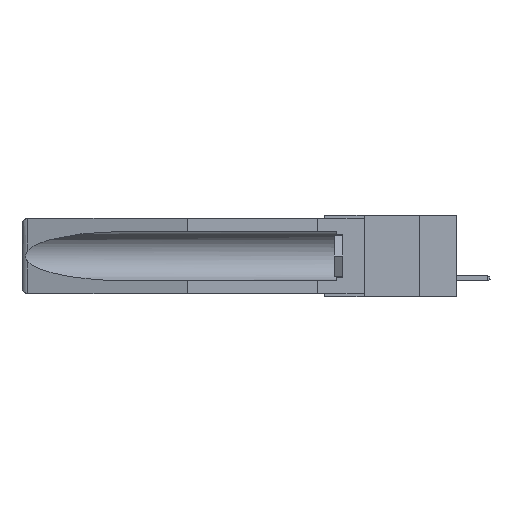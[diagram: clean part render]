
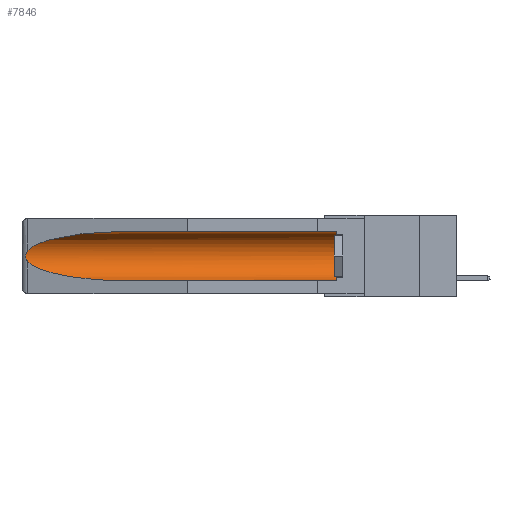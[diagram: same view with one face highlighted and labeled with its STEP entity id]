
A CAD part, left-side view. The second image highlights one B-rep face of the part: STEP entity #7846.
In plain terms, the highlighted cylindrical face has radius 2.857 mm (diameter 5.715 mm), a partial arc.
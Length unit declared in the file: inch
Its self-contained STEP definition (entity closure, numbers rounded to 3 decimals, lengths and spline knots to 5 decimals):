
#14 = CYLINDRICAL_SURFACE ( 'NONE', #1620, 0.1125 ) ;
#582 = CARTESIAN_POINT ( 'NONE',  ( 0.155, -0.30754, -0.284 ) ) ;
#1620 = AXIS2_PLACEMENT_3D ( 'NONE', #8060, #27274, #1698 ) ;
#1633 = CARTESIAN_POINT ( 'NONE',  ( 0.155, 0.126, -0.059 ) ) ;
#1698 = DIRECTION ( 'NONE',  ( 0., 0., 1. ) ) ;
#1851 = CARTESIAN_POINT ( 'NONE',  ( 0.26537, 1.52718, -0.14972 ) ) ;
#2021 = CARTESIAN_POINT ( 'NONE',  ( 0.2675, 1.53308, -0.17534 ) ) ;
#3141 = CARTESIAN_POINT ( 'NONE',  ( 0.26537, 1.52718, -0.19328 ) ) ;
#3952 = CARTESIAN_POINT ( 'NONE',  ( 0.26597, 1.5296, -0.19026 ) ) ;
#4129 = EDGE_CURVE ( 'NONE', #7265, #11339, #20582, .T. ) ;
#4150 = CARTESIAN_POINT ( 'NONE',  ( 0.26537, 1.52718, -0.14972 ) ) ;
#4466 = VERTEX_POINT ( 'NONE', #5350 ) ;
#5350 = CARTESIAN_POINT ( 'NONE',  ( 0.26537, 1.52718, -0.14972 ) ) ;
#5520 = EDGE_CURVE ( 'NONE', #24742, #11339, #21461, .T. ) ;
#6110 = AXIS2_PLACEMENT_3D ( 'NONE', #10909, #21558, #17171 ) ;
#6235 = CARTESIAN_POINT ( 'NONE',  ( 0.26537, 1.52718, -0.19328 ) ) ;
#6676 = ORIENTED_EDGE ( 'NONE', *, *, #16037, .T. ) ;
#6684 = ORIENTED_EDGE ( 'NONE', *, *, #20592, .T. ) ;
#7265 = VERTEX_POINT ( 'NONE', #25943 ) ;
#7846 = ADVANCED_FACE ( 'NONE', ( #17055 ), #14, .F. ) ;
#8060 = CARTESIAN_POINT ( 'NONE',  ( 0.155, -0.30754, -0.1715 ) ) ;
#8116 = DIRECTION ( 'NONE',  ( 0., 1., 0. ) ) ;
#8688 = CARTESIAN_POINT ( 'NONE',  ( 0.155, 1.07973, -0.284 ) ) ;
#9482 =( BOUNDED_CURVE ( )  B_SPLINE_CURVE ( 3, ( #14633, #25220, #20997, #4150 ),
 .UNSPECIFIED., .F., .F. ) 
 B_SPLINE_CURVE_WITH_KNOTS ( ( 4, 4 ),
 ( 4.71239, 6.08839 ),
 .UNSPECIFIED. ) 
 CURVE ( )  GEOMETRIC_REPRESENTATION_ITEM ( )  RATIONAL_B_SPLINE_CURVE ( ( 1., 0.848, 0.848, 1. ) ) 
 REPRESENTATION_ITEM ( '' )  );
#10348 = CARTESIAN_POINT ( 'NONE',  ( 0.155, -0.30754, -0.059 ) ) ;
#10535 = CARTESIAN_POINT ( 'NONE',  ( 0.2673, 1.53269, -0.17917 ) ) ;
#10909 = CARTESIAN_POINT ( 'NONE',  ( 0.155, 0.126, -0.1715 ) ) ;
#10919 = CARTESIAN_POINT ( 'NONE',  ( 0.26537, 1.52718, -0.19328 ) ) ;
#11054 = CIRCLE ( 'NONE', #6110, 0.1125 ) ;
#11339 = VERTEX_POINT ( 'NONE', #8688 ) ;
#13080 = CARTESIAN_POINT ( 'NONE',  ( 0.155, 1.07973, -0.284 ) ) ;
#13252 = B_SPLINE_CURVE_WITH_KNOTS ( 'NONE', 3,
 ( #1851, #19094, #16762, #19007, #23263, #2021, #10535, #18917, #3952, #6235 ),
 .UNSPECIFIED., .F., .F.,
 ( 4, 2, 2, 2, 4 ),
 ( 0., 0.00029, 0.00058, 0.00087, 0.00117 ),
 .UNSPECIFIED. ) ;
#13454 = EDGE_LOOP ( 'NONE', ( #22214, #6676, #24515, #17162, #6684, #22376 ) ) ;
#14633 = CARTESIAN_POINT ( 'NONE',  ( 0.155, 1.07973, -0.059 ) ) ;
#15475 = VERTEX_POINT ( 'NONE', #1633 ) ;
#16037 = EDGE_CURVE ( 'NONE', #4466, #24742, #13252, .T. ) ;
#16142 = EDGE_CURVE ( 'NONE', #15475, #20311, #24009, .T. ) ;
#16762 = CARTESIAN_POINT ( 'NONE',  ( 0.26654, 1.53092, -0.15636 ) ) ;
#17055 = FACE_OUTER_BOUND ( 'NONE', #13454, .T. ) ;
#17162 = ORIENTED_EDGE ( 'NONE', *, *, #4129, .F. ) ;
#17171 = DIRECTION ( 'NONE',  ( 0., 0., 1. ) ) ;
#18917 = CARTESIAN_POINT ( 'NONE',  ( 0.26655, 1.53094, -0.18657 ) ) ;
#19007 = CARTESIAN_POINT ( 'NONE',  ( 0.2673, 1.5327, -0.16383 ) ) ;
#19094 = CARTESIAN_POINT ( 'NONE',  ( 0.26597, 1.52961, -0.15275 ) ) ;
#19510 = DIRECTION ( 'NONE',  ( 0., 1., 0. ) ) ;
#20311 = VERTEX_POINT ( 'NONE', #20529 ) ;
#20529 = CARTESIAN_POINT ( 'NONE',  ( 0.155, 1.07973, -0.059 ) ) ;
#20582 = LINE ( 'NONE', #582, #24932 ) ;
#20592 = EDGE_CURVE ( 'NONE', #7265, #15475, #11054, .T. ) ;
#20997 = CARTESIAN_POINT ( 'NONE',  ( 0.25451, 1.48313, -0.09465 ) ) ;
#21461 =( BOUNDED_CURVE ( )  B_SPLINE_CURVE ( 3, ( #10919, #25779, #23829, #13080 ),
 .UNSPECIFIED., .F., .F. ) 
 B_SPLINE_CURVE_WITH_KNOTS ( ( 4, 4 ),
 ( 0.1948, 1.5708 ),
 .UNSPECIFIED. ) 
 CURVE ( )  GEOMETRIC_REPRESENTATION_ITEM ( )  RATIONAL_B_SPLINE_CURVE ( ( 1., 0.848, 0.848, 1. ) ) 
 REPRESENTATION_ITEM ( '' )  );
#21558 = DIRECTION ( 'NONE',  ( 0., -1., 0. ) ) ;
#21987 = VECTOR ( 'NONE', #8116, 39.37008 ) ;
#22214 = ORIENTED_EDGE ( 'NONE', *, *, #26323, .T. ) ;
#22376 = ORIENTED_EDGE ( 'NONE', *, *, #16142, .T. ) ;
#23263 = CARTESIAN_POINT ( 'NONE',  ( 0.2675, 1.53308, -0.16763 ) ) ;
#23829 = CARTESIAN_POINT ( 'NONE',  ( 0.21114, 1.30732, -0.284 ) ) ;
#24009 = LINE ( 'NONE', #10348, #21987 ) ;
#24515 = ORIENTED_EDGE ( 'NONE', *, *, #5520, .T. ) ;
#24742 = VERTEX_POINT ( 'NONE', #3141 ) ;
#24932 = VECTOR ( 'NONE', #19510, 39.37008 ) ;
#25220 = CARTESIAN_POINT ( 'NONE',  ( 0.21114, 1.30732, -0.059 ) ) ;
#25779 = CARTESIAN_POINT ( 'NONE',  ( 0.25451, 1.48313, -0.24835 ) ) ;
#25943 = CARTESIAN_POINT ( 'NONE',  ( 0.155, 0.126, -0.284 ) ) ;
#26323 = EDGE_CURVE ( 'NONE', #20311, #4466, #9482, .T. ) ;
#27274 = DIRECTION ( 'NONE',  ( 0., 1., 0. ) ) ;
